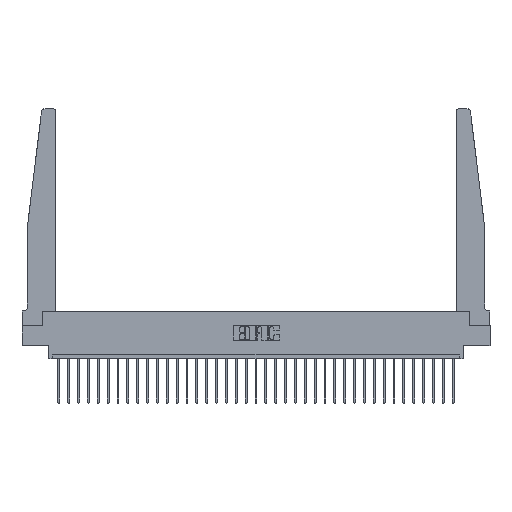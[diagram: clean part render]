
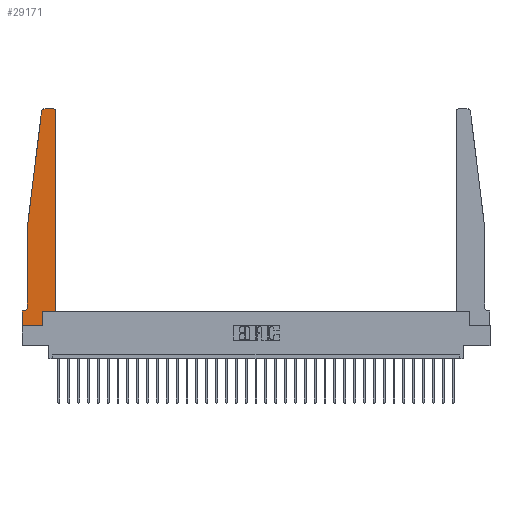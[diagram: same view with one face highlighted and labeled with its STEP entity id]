
A CAD part, top view. The second image highlights one B-rep face of the part: STEP entity #29171.
In plain terms, the highlighted planar face has unit normal (0, 0, 1).
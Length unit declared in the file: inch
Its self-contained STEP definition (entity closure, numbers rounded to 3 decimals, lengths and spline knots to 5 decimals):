
#490 = CARTESIAN_POINT ( 'NONE',  ( 0.395, 2.72, 0.37 ) ) ;
#620 = EDGE_CURVE ( 'NONE', #1423, #10684, #3537, .T. ) ;
#1199 = DIRECTION ( 'NONE',  ( 1., 0., 0. ) ) ;
#1414 = EDGE_CURVE ( 'NONE', #6650, #9083, #3385, .T. ) ;
#1423 = VERTEX_POINT ( 'NONE', #30658 ) ;
#1478 = VERTEX_POINT ( 'NONE', #18739 ) ;
#1495 = LINE ( 'NONE', #6178, #12438 ) ;
#1696 = ORIENTED_EDGE ( 'NONE', *, *, #620, .T. ) ;
#1809 = AXIS2_PLACEMENT_3D ( 'NONE', #27373, #8273, #20471 ) ;
#2738 = DIRECTION ( 'NONE',  ( 1., 0., 0. ) ) ;
#3162 = DIRECTION ( 'NONE',  ( 0., 0., -1. ) ) ;
#3385 = CIRCLE ( 'NONE', #1809, 0.03 ) ;
#3537 = LINE ( 'NONE', #5575, #6447 ) ;
#4045 = ORIENTED_EDGE ( 'NONE', *, *, #28877, .T. ) ;
#4332 = EDGE_CURVE ( 'NONE', #27901, #1478, #22611, .T. ) ;
#4375 = ORIENTED_EDGE ( 'NONE', *, *, #15745, .T. ) ;
#4386 = DIRECTION ( 'NONE',  ( 0., 1., 0. ) ) ;
#4604 = VERTEX_POINT ( 'NONE', #7401 ) ;
#4903 = VECTOR ( 'NONE', #10154, 39.37008 ) ;
#5024 = DIRECTION ( 'NONE',  ( 0., 0., 1. ) ) ;
#5051 = ORIENTED_EDGE ( 'NONE', *, *, #1414, .T. ) ;
#5392 = PLANE ( 'NONE',  #9383 ) ;
#5575 = CARTESIAN_POINT ( 'NONE',  ( 0.425, 0.18, 0.37 ) ) ;
#6178 = CARTESIAN_POINT ( 'NONE',  ( 0.065, 1.25, 0.37 ) ) ;
#6447 = VECTOR ( 'NONE', #1199, 39.37008 ) ;
#6650 = VERTEX_POINT ( 'NONE', #27390 ) ;
#7182 = CARTESIAN_POINT ( 'NONE',  ( 0.425, 2.72, 0.37 ) ) ;
#7401 = CARTESIAN_POINT ( 'NONE',  ( 0.395, 2.75, 0.37 ) ) ;
#7761 = CARTESIAN_POINT ( 'NONE',  ( 0.425, 0.18, 0.37 ) ) ;
#7791 = LINE ( 'NONE', #27057, #4903 ) ;
#7824 = LINE ( 'NONE', #24578, #19654 ) ;
#8273 = DIRECTION ( 'NONE',  ( 0., 0., 1. ) ) ;
#8663 = CARTESIAN_POINT ( 'NONE',  ( 0.2605, 0.18, 0.37 ) ) ;
#9083 = VERTEX_POINT ( 'NONE', #11662 ) ;
#9357 = VERTEX_POINT ( 'NONE', #24932 ) ;
#9383 = AXIS2_PLACEMENT_3D ( 'NONE', #10256, #17435, #2738 ) ;
#10154 = DIRECTION ( 'NONE',  ( -1., 0., 0. ) ) ;
#10251 = CARTESIAN_POINT ( 'NONE',  ( 0.25, 2.75, 0.37 ) ) ;
#10256 = CARTESIAN_POINT ( 'NONE',  ( 0., 0.1875, 0.37 ) ) ;
#10481 = ORIENTED_EDGE ( 'NONE', *, *, #29946, .T. ) ;
#10684 = VERTEX_POINT ( 'NONE', #7761 ) ;
#11044 = DIRECTION ( 'NONE',  ( 0., -1., 0. ) ) ;
#11449 = LINE ( 'NONE', #25222, #17263 ) ;
#11662 = CARTESIAN_POINT ( 'NONE',  ( 0.24675, 2.72367, 0.37 ) ) ;
#12164 = ORIENTED_EDGE ( 'NONE', *, *, #21449, .T. ) ;
#12438 = VECTOR ( 'NONE', #11044, 39.37008 ) ;
#12606 = DIRECTION ( 'NONE',  ( -1., 0., 0. ) ) ;
#12777 = CIRCLE ( 'NONE', #19259, 0.05 ) ;
#14856 = DIRECTION ( 'NONE',  ( -0.122, -0.992, 0. ) ) ;
#14942 = ORIENTED_EDGE ( 'NONE', *, *, #18888, .T. ) ;
#15143 = VERTEX_POINT ( 'NONE', #20319 ) ;
#15745 = EDGE_CURVE ( 'NONE', #9357, #15143, #12777, .T. ) ;
#15968 = EDGE_CURVE ( 'NONE', #10684, #18228, #11449, .T. ) ;
#16020 = CARTESIAN_POINT ( 'NONE',  ( 0., 0., 0.37 ) ) ;
#16397 = ORIENTED_EDGE ( 'NONE', *, *, #23282, .T. ) ;
#16870 = ORIENTED_EDGE ( 'NONE', *, *, #15968, .T. ) ;
#17197 = CARTESIAN_POINT ( 'NONE',  ( 0.065, 1.25, 0.37 ) ) ;
#17263 = VECTOR ( 'NONE', #4386, 39.37008 ) ;
#17435 = DIRECTION ( 'NONE',  ( 0., 0., 1. ) ) ;
#18228 = VERTEX_POINT ( 'NONE', #7182 ) ;
#18366 = ORIENTED_EDGE ( 'NONE', *, *, #28240, .T. ) ;
#18739 = CARTESIAN_POINT ( 'NONE',  ( 0., 0., 0.37 ) ) ;
#18888 = EDGE_CURVE ( 'NONE', #18228, #4604, #26809, .T. ) ;
#19176 = CARTESIAN_POINT ( 'NONE',  ( 0., 0., 0.37 ) ) ;
#19259 = AXIS2_PLACEMENT_3D ( 'NONE', #24914, #3162, #29474 ) ;
#19267 = CARTESIAN_POINT ( 'NONE',  ( 0.2605, 0., 0.37 ) ) ;
#19570 = VECTOR ( 'NONE', #22895, 39.37008 ) ;
#19654 = VECTOR ( 'NONE', #14856, 39.37008 ) ;
#19684 = VECTOR ( 'NONE', #28740, 39.37008 ) ;
#20319 = CARTESIAN_POINT ( 'NONE',  ( 0.015, 0.1875, 0.37 ) ) ;
#20471 = DIRECTION ( 'NONE',  ( 1., 0., 0. ) ) ;
#21449 = EDGE_CURVE ( 'NONE', #22477, #9357, #1495, .T. ) ;
#21531 = LINE ( 'NONE', #19176, #19684 ) ;
#22019 = VECTOR ( 'NONE', #27776, 39.37008 ) ;
#22253 = CARTESIAN_POINT ( 'NONE',  ( 0., 0.1875, 0.37 ) ) ;
#22407 = EDGE_LOOP ( 'NONE', ( #16397, #5051, #18366, #12164, #4375, #10481, #27403, #4045, #24919, #1696, #16870, #14942 ) ) ;
#22477 = VERTEX_POINT ( 'NONE', #17197 ) ;
#22611 = LINE ( 'NONE', #16020, #22019 ) ;
#22895 = DIRECTION ( 'NONE',  ( 0., 1., 0. ) ) ;
#23282 = EDGE_CURVE ( 'NONE', #4604, #6650, #26383, .T. ) ;
#23804 = AXIS2_PLACEMENT_3D ( 'NONE', #490, #5024, #26318 ) ;
#24187 = FACE_OUTER_BOUND ( 'NONE', #22407, .T. ) ;
#24517 = VECTOR ( 'NONE', #12606, 39.37008 ) ;
#24578 = CARTESIAN_POINT ( 'NONE',  ( 0.065, 1.25, 0.37 ) ) ;
#24914 = CARTESIAN_POINT ( 'NONE',  ( 0.015, 0.2375, 0.37 ) ) ;
#24919 = ORIENTED_EDGE ( 'NONE', *, *, #26188, .T. ) ;
#24932 = CARTESIAN_POINT ( 'NONE',  ( 0.065, 0.2375, 0.37 ) ) ;
#25222 = CARTESIAN_POINT ( 'NONE',  ( 0.425, 0.18, 0.37 ) ) ;
#25570 = LINE ( 'NONE', #8663, #19570 ) ;
#26188 = EDGE_CURVE ( 'NONE', #30423, #1423, #25570, .T. ) ;
#26318 = DIRECTION ( 'NONE',  ( 1., 0., 0. ) ) ;
#26383 = LINE ( 'NONE', #10251, #24517 ) ;
#26809 = CIRCLE ( 'NONE', #23804, 0.03 ) ;
#27057 = CARTESIAN_POINT ( 'NONE',  ( 0.065, 0.1875, 0.37 ) ) ;
#27373 = CARTESIAN_POINT ( 'NONE',  ( 0.27653, 2.72, 0.37 ) ) ;
#27390 = CARTESIAN_POINT ( 'NONE',  ( 0.27653, 2.75, 0.37 ) ) ;
#27403 = ORIENTED_EDGE ( 'NONE', *, *, #4332, .T. ) ;
#27776 = DIRECTION ( 'NONE',  ( 0., -1., 0. ) ) ;
#27901 = VERTEX_POINT ( 'NONE', #22253 ) ;
#28240 = EDGE_CURVE ( 'NONE', #9083, #22477, #7824, .T. ) ;
#28740 = DIRECTION ( 'NONE',  ( 1., 0., 0. ) ) ;
#28877 = EDGE_CURVE ( 'NONE', #1478, #30423, #21531, .T. ) ;
#29171 = ADVANCED_FACE ( 'NONE', ( #24187 ), #5392, .T. ) ;
#29474 = DIRECTION ( 'NONE',  ( -1., 0., 0. ) ) ;
#29946 = EDGE_CURVE ( 'NONE', #15143, #27901, #7791, .T. ) ;
#30423 = VERTEX_POINT ( 'NONE', #19267 ) ;
#30658 = CARTESIAN_POINT ( 'NONE',  ( 0.2605, 0.18, 0.37 ) ) ;
